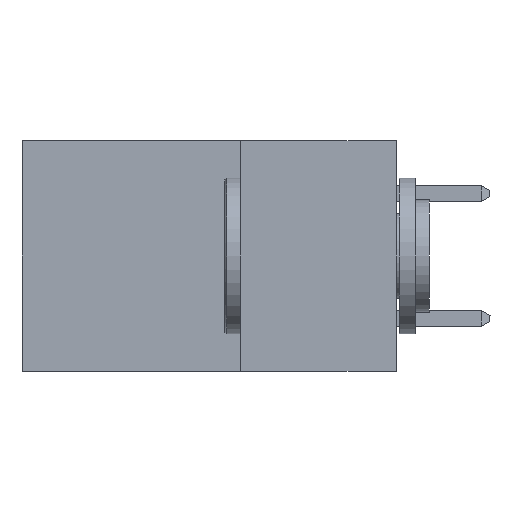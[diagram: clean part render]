
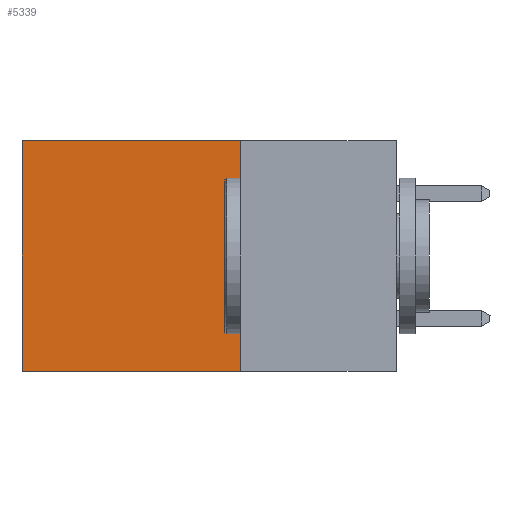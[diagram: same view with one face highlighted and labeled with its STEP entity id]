
A CAD part, left-side view. The second image highlights one B-rep face of the part: STEP entity #5339.
In plain terms, the highlighted planar face has unit normal (-1, 0, 0).
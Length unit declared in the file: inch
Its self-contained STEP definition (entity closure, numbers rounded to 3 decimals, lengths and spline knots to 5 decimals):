
#365 = EDGE_LOOP ( 'NONE', ( #1192, #5971, #8845, #7813 ) ) ;
#457 = DIRECTION ( 'NONE',  ( 0., 0., -1. ) ) ;
#930 = LINE ( 'NONE', #6089, #4922 ) ;
#943 = EDGE_CURVE ( 'NONE', #7993, #5449, #9102, .T. ) ;
#1136 = CARTESIAN_POINT ( 'NONE',  ( 0.298, 0.6, 0. ) ) ;
#1192 = ORIENTED_EDGE ( 'NONE', *, *, #943, .T. ) ;
#1551 = DIRECTION ( 'NONE',  ( 1., 0., 0. ) ) ;
#2378 = EDGE_CURVE ( 'NONE', #4988, #7993, #5983, .T. ) ;
#3383 = VERTEX_POINT ( 'NONE', #9532 ) ;
#3678 = VECTOR ( 'NONE', #7594, 39.37008 ) ;
#4459 = CARTESIAN_POINT ( 'NONE',  ( 0.298, 0.25, 0. ) ) ;
#4465 = EDGE_CURVE ( 'NONE', #3383, #5449, #930, .T. ) ;
#4922 = VECTOR ( 'NONE', #7694, 39.37008 ) ;
#4988 = VERTEX_POINT ( 'NONE', #4459 ) ;
#5061 = CARTESIAN_POINT ( 'NONE',  ( 0.298, 0.25, 0. ) ) ;
#5339 = ADVANCED_FACE ( 'NONE', ( #6057 ), #7350, .F. ) ;
#5449 = VERTEX_POINT ( 'NONE', #6625 ) ;
#5763 = EDGE_CURVE ( 'NONE', #4988, #3383, #9526, .T. ) ;
#5971 = ORIENTED_EDGE ( 'NONE', *, *, #4465, .F. ) ;
#5983 = LINE ( 'NONE', #5061, #3678 ) ;
#6057 = FACE_OUTER_BOUND ( 'NONE', #365, .T. ) ;
#6089 = CARTESIAN_POINT ( 'NONE',  ( 0.298, 0.25, -0.37 ) ) ;
#6625 = CARTESIAN_POINT ( 'NONE',  ( 0.298, 0.6, -0.37 ) ) ;
#7350 = PLANE ( 'NONE',  #10516 ) ;
#7594 = DIRECTION ( 'NONE',  ( 0., 1., 0. ) ) ;
#7694 = DIRECTION ( 'NONE',  ( 0., 1., 0. ) ) ;
#7709 = VECTOR ( 'NONE', #9295, 39.37008 ) ;
#7813 = ORIENTED_EDGE ( 'NONE', *, *, #2378, .T. ) ;
#7993 = VERTEX_POINT ( 'NONE', #8113 ) ;
#8113 = CARTESIAN_POINT ( 'NONE',  ( 0.298, 0.6, 0. ) ) ;
#8644 = CARTESIAN_POINT ( 'NONE',  ( 0.298, 0.25, 0. ) ) ;
#8845 = ORIENTED_EDGE ( 'NONE', *, *, #5763, .F. ) ;
#9102 = LINE ( 'NONE', #1136, #7709 ) ;
#9136 = VECTOR ( 'NONE', #457, 39.37008 ) ;
#9295 = DIRECTION ( 'NONE',  ( 0., 0., -1. ) ) ;
#9526 = LINE ( 'NONE', #8644, #9136 ) ;
#9532 = CARTESIAN_POINT ( 'NONE',  ( 0.298, 0.25, -0.37 ) ) ;
#9787 = CARTESIAN_POINT ( 'NONE',  ( 0.298, 0.25, 0. ) ) ;
#9895 = DIRECTION ( 'NONE',  ( 0., 0., -1. ) ) ;
#10516 = AXIS2_PLACEMENT_3D ( 'NONE', #9787, #1551, #9895 ) ;
